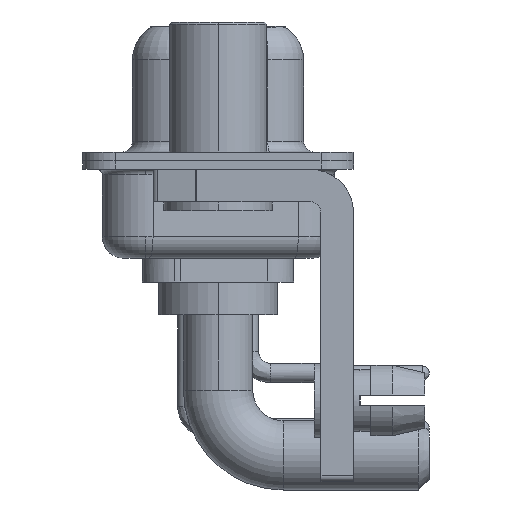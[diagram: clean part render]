
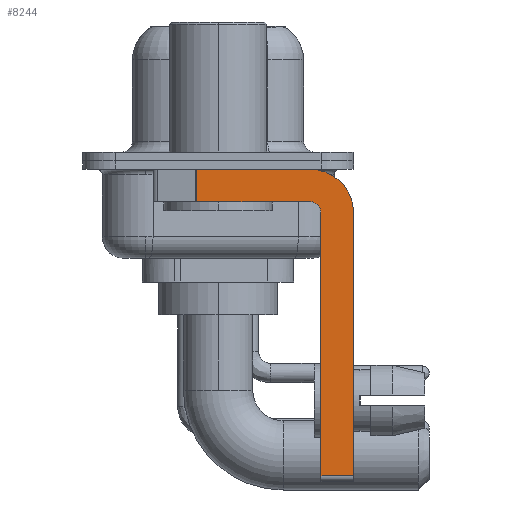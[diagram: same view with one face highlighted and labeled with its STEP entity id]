
A CAD part, left-side view. The second image highlights one B-rep face of the part: STEP entity #8244.
In plain terms, the highlighted planar face has unit normal (-1, 0, 0).
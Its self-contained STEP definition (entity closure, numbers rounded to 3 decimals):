
#565 = VECTOR ( 'NONE', #1750, 1000. ) ;
#990 = DIRECTION ( 'NONE',  ( 1., 0., 0. ) ) ;
#1263 = ORIENTED_EDGE ( 'NONE', *, *, #17468, .F. ) ;
#1365 = DIRECTION ( 'NONE',  ( 0., 0., -1. ) ) ;
#1750 = DIRECTION ( 'NONE',  ( 0., 0., -1. ) ) ;
#1824 = DIRECTION ( 'NONE',  ( -1., 0., 0. ) ) ;
#2678 = CARTESIAN_POINT ( 'NONE',  ( -2.9, -6.25, -14.55 ) ) ;
#3087 = EDGE_CURVE ( 'NONE', #22142, #13848, #9398, .T. ) ;
#3457 = CARTESIAN_POINT ( 'NONE',  ( -2.9, -4.25, -2.4 ) ) ;
#3765 = DIRECTION ( 'NONE',  ( 0., -1., 0. ) ) ;
#4137 = AXIS2_PLACEMENT_3D ( 'NONE', #24108, #14568, #4501 ) ;
#4501 = DIRECTION ( 'NONE',  ( 0., 0., -1. ) ) ;
#4547 = VERTEX_POINT ( 'NONE', #2678 ) ;
#5088 = CARTESIAN_POINT ( 'NONE',  ( -2.9, -6.25, -2.4 ) ) ;
#5526 = DIRECTION ( 'NONE',  ( 0., 1., 0. ) ) ;
#6258 = ORIENTED_EDGE ( 'NONE', *, *, #15657, .T. ) ;
#6974 = FACE_OUTER_BOUND ( 'NONE', #19484, .T. ) ;
#7064 = LINE ( 'NONE', #22786, #19266 ) ;
#7291 = LINE ( 'NONE', #5088, #21655 ) ;
#7854 = CIRCLE ( 'NONE', #4137, 2. ) ;
#7973 = VERTEX_POINT ( 'NONE', #13206 ) ;
#8244 = ADVANCED_FACE ( 'NONE', ( #6974 ), #18958, .F. ) ;
#8246 = VERTEX_POINT ( 'NONE', #16893 ) ;
#8901 = CIRCLE ( 'NONE', #22898, 0.5 ) ;
#9165 = CARTESIAN_POINT ( 'NONE',  ( -2.9, -4.75, -14.8 ) ) ;
#9398 = LINE ( 'NONE', #23202, #12790 ) ;
#9468 = CARTESIAN_POINT ( 'NONE',  ( -2.9, -4.25, -2.4 ) ) ;
#10802 = EDGE_CURVE ( 'NONE', #7973, #13848, #23199, .T. ) ;
#10978 = DIRECTION ( 'NONE',  ( 0., 0., 1. ) ) ;
#11281 = VECTOR ( 'NONE', #10978, 1000. ) ;
#11545 = DIRECTION ( 'NONE',  ( 0., 0., 1. ) ) ;
#11623 = EDGE_CURVE ( 'NONE', #17145, #4547, #7291, .T. ) ;
#12790 = VECTOR ( 'NONE', #5526, 1000. ) ;
#12996 = DIRECTION ( 'NONE',  ( 0., -1., 0. ) ) ;
#13206 = CARTESIAN_POINT ( 'NONE',  ( -2.9, 0.978, -0.4 ) ) ;
#13848 = VERTEX_POINT ( 'NONE', #22075 ) ;
#14059 = ORIENTED_EDGE ( 'NONE', *, *, #15019, .F. ) ;
#14568 = DIRECTION ( 'NONE',  ( 1., 0., 0. ) ) ;
#14717 = CARTESIAN_POINT ( 'NONE',  ( -2.9, -4.75, -2.4 ) ) ;
#15019 = EDGE_CURVE ( 'NONE', #7973, #8246, #7064, .T. ) ;
#15657 = EDGE_CURVE ( 'NONE', #25369, #4547, #23130, .T. ) ;
#15784 = VERTEX_POINT ( 'NONE', #14717 ) ;
#16238 = AXIS2_PLACEMENT_3D ( 'NONE', #3457, #990, #1365 ) ;
#16242 = ORIENTED_EDGE ( 'NONE', *, *, #11623, .F. ) ;
#16787 = CARTESIAN_POINT ( 'NONE',  ( -2.9, -6.25, -2.4 ) ) ;
#16893 = CARTESIAN_POINT ( 'NONE',  ( -2.9, -4.25, -0.4 ) ) ;
#17145 = VERTEX_POINT ( 'NONE', #16787 ) ;
#17468 = EDGE_CURVE ( 'NONE', #8246, #17145, #7854, .T. ) ;
#18078 = CARTESIAN_POINT ( 'NONE',  ( -2.9, -4.75, -14.55 ) ) ;
#18879 = VECTOR ( 'NONE', #3765, 1000. ) ;
#18958 = PLANE ( 'NONE',  #16238 ) ;
#19149 = DIRECTION ( 'NONE',  ( 0., 0., -1. ) ) ;
#19266 = VECTOR ( 'NONE', #12996, 1000. ) ;
#19484 = EDGE_LOOP ( 'NONE', ( #14059, #19726, #20732, #25525, #24412, #6258, #16242, #1263 ) ) ;
#19726 = ORIENTED_EDGE ( 'NONE', *, *, #10802, .T. ) ;
#20732 = ORIENTED_EDGE ( 'NONE', *, *, #3087, .F. ) ;
#21135 = CARTESIAN_POINT ( 'NONE',  ( -2.9, 0.978, -1.9 ) ) ;
#21448 = CARTESIAN_POINT ( 'NONE',  ( -2.9, -4.25, -14.55 ) ) ;
#21655 = VECTOR ( 'NONE', #19149, 1000. ) ;
#21959 = EDGE_CURVE ( 'NONE', #25369, #15784, #23209, .T. ) ;
#22075 = CARTESIAN_POINT ( 'NONE',  ( -2.9, 0.978, -1.9 ) ) ;
#22142 = VERTEX_POINT ( 'NONE', #25263 ) ;
#22786 = CARTESIAN_POINT ( 'NONE',  ( -2.9, 3., -0.4 ) ) ;
#22898 = AXIS2_PLACEMENT_3D ( 'NONE', #9468, #1824, #11545 ) ;
#23130 = LINE ( 'NONE', #21448, #18879 ) ;
#23199 = LINE ( 'NONE', #21135, #565 ) ;
#23202 = CARTESIAN_POINT ( 'NONE',  ( -2.9, -4.25, -1.9 ) ) ;
#23209 = LINE ( 'NONE', #9165, #11281 ) ;
#24108 = CARTESIAN_POINT ( 'NONE',  ( -2.9, -4.25, -2.4 ) ) ;
#24412 = ORIENTED_EDGE ( 'NONE', *, *, #21959, .F. ) ;
#24416 = EDGE_CURVE ( 'NONE', #15784, #22142, #8901, .T. ) ;
#25263 = CARTESIAN_POINT ( 'NONE',  ( -2.9, -4.25, -1.9 ) ) ;
#25369 = VERTEX_POINT ( 'NONE', #18078 ) ;
#25525 = ORIENTED_EDGE ( 'NONE', *, *, #24416, .F. ) ;
